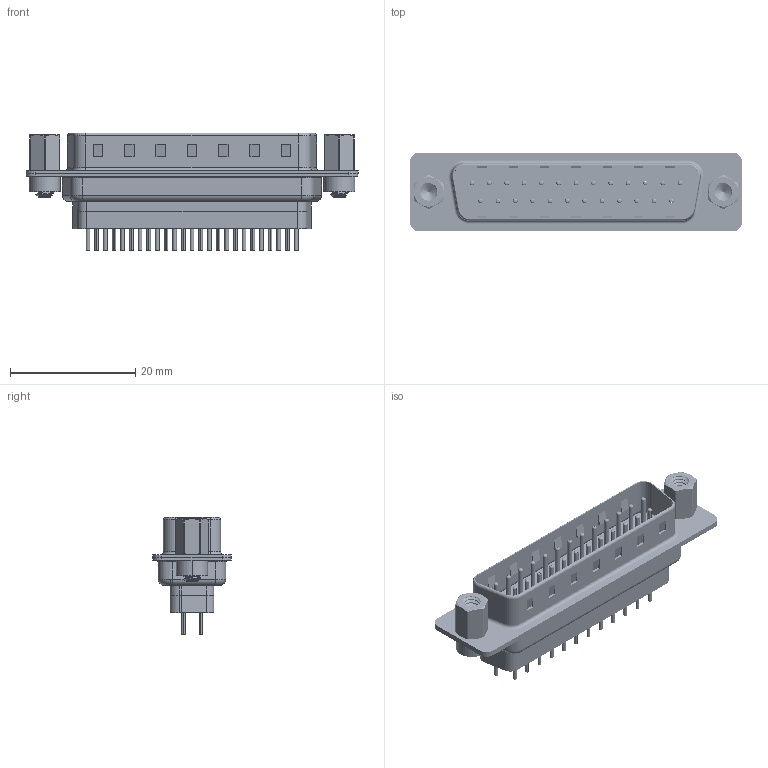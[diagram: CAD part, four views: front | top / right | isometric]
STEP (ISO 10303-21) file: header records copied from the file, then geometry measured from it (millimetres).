
FILE_DESCRIPTION (( 'STEP AP203' ), '1' );
FILE_NAME ('627-025-228-263.STEP', '2020-07-21T16:47:38', ( '' ), ( '' ), 'SwSTEP 2.0', 'SolidWorks 2020', '' );
FILE_SCHEMA (( 'CONFIG_CONTROL_DESIGN' ));
Length unit declared in the file: millimetre
Products named in the file (8): 627 Housing_25 FF; 627 Shell Front_25 Contacts; 627-025-228-263; 627 Shell Rear_25 Contacts; 627 Contact Row 2_28L; 627 Contact Row 1_28L; 627 4-40 Hex Standoff; 627 4-40 Threaded Rivet
Assembly tree (32 placements, depth 2):
  627-025-228-263
    627 Housing_25 FF
    627 Shell Front_25 Contacts
    627 Shell Rear_25 Contacts
    627 Contact Row 1_28L  x13
    627 Contact Row 2_28L  x12
    627 4-40 Threaded Rivet  x2
    627 4-40 Hex Standoff  x2
Bounding box: 53 x 12.6 x 18.8 mm (x, y, z)
Volume: 3485.1 mm3; surface area: 9396.6 mm2
Topology: 33 solids, 33 shells, 3009 faces, 7893 edges, 4911 vertices
Faces by surface type: cylinder 1187, plane 799, torus 725, cone 280, bspline 18
Entity records: 31615 total; most frequent: CARTESIAN_POINT 8986, DIRECTION 4656, ORIENTED_EDGE 4276, EDGE_CURVE 2138, AXIS2_PLACEMENT_3D 1845, VERTEX_POINT 1370, EDGE_LOOP 1048, CIRCLE 974
